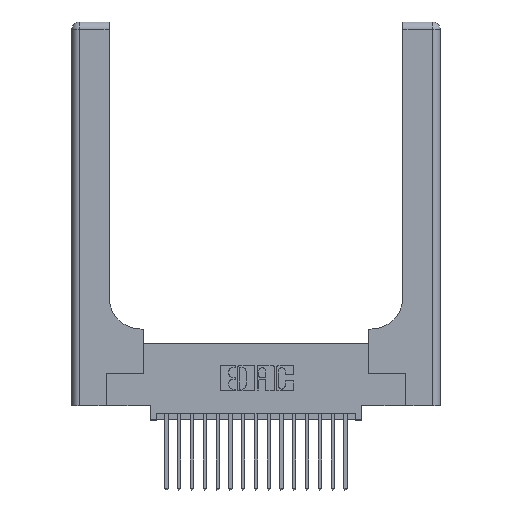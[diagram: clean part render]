
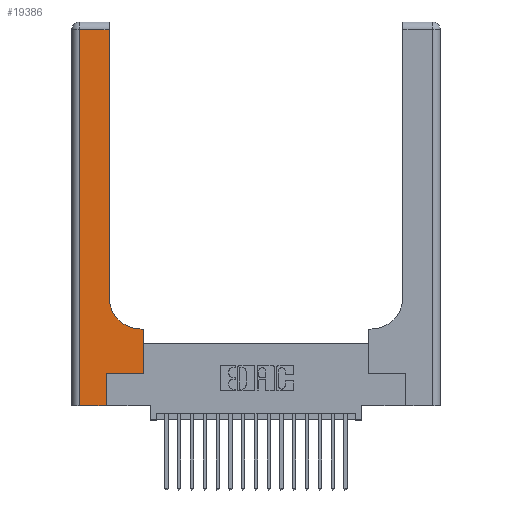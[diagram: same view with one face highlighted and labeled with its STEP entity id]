
A CAD part, top view. The second image highlights one B-rep face of the part: STEP entity #19386.
In plain terms, the highlighted planar face has unit normal (0, 0, 1).
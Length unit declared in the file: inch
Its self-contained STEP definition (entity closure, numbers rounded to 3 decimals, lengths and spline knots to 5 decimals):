
#181 = DIRECTION ( 'NONE',  ( 1., 0., 0. ) ) ;
#705 = LINE ( 'NONE', #16932, #8819 ) ;
#748 = VERTEX_POINT ( 'NONE', #1875 ) ;
#1080 = EDGE_CURVE ( 'NONE', #4931, #9926, #705, .T. ) ;
#1143 = DIRECTION ( 'NONE',  ( 0., 1., 0. ) ) ;
#1218 = ORIENTED_EDGE ( 'NONE', *, *, #17493, .T. ) ;
#1386 = VERTEX_POINT ( 'NONE', #12936 ) ;
#1822 = VECTOR ( 'NONE', #181, 39.37008 ) ;
#1875 = CARTESIAN_POINT ( 'NONE',  ( 0.2915, 2.94, 0.37 ) ) ;
#2050 = LINE ( 'NONE', #8583, #17561 ) ;
#3227 = EDGE_CURVE ( 'NONE', #7083, #1386, #7642, .T. ) ;
#3342 = VECTOR ( 'NONE', #7728, 39.37008 ) ;
#3716 = AXIS2_PLACEMENT_3D ( 'NONE', #9693, #17156, #11349 ) ;
#3732 = LINE ( 'NONE', #12469, #11854 ) ;
#3959 = AXIS2_PLACEMENT_3D ( 'NONE', #14733, #5091, #16300 ) ;
#4046 = CIRCLE ( 'NONE', #3959, 0.25 ) ;
#4320 = CARTESIAN_POINT ( 'NONE',  ( 0.2915, 3., 0.37 ) ) ;
#4522 = VERTEX_POINT ( 'NONE', #17471 ) ;
#4611 = ORIENTED_EDGE ( 'NONE', *, *, #19188, .T. ) ;
#4773 = CARTESIAN_POINT ( 'NONE',  ( 0., 2.94, 0.37 ) ) ;
#4931 = VERTEX_POINT ( 'NONE', #13647 ) ;
#5091 = DIRECTION ( 'NONE',  ( 0., 0., -1. ) ) ;
#5169 = ORIENTED_EDGE ( 'NONE', *, *, #17136, .T. ) ;
#5194 = ORIENTED_EDGE ( 'NONE', *, *, #13864, .T. ) ;
#5975 = LINE ( 'NONE', #16312, #18178 ) ;
#6339 = VERTEX_POINT ( 'NONE', #17138 ) ;
#7083 = VERTEX_POINT ( 'NONE', #10595 ) ;
#7498 = VECTOR ( 'NONE', #17559, 39.37008 ) ;
#7582 = DIRECTION ( 'NONE',  ( 0., 1., 0. ) ) ;
#7642 = LINE ( 'NONE', #8722, #3342 ) ;
#7728 = DIRECTION ( 'NONE',  ( 1., 0., 0. ) ) ;
#8287 = VERTEX_POINT ( 'NONE', #20000 ) ;
#8354 = DIRECTION ( 'NONE',  ( 0., -1., 0. ) ) ;
#8583 = CARTESIAN_POINT ( 'NONE',  ( 0.269, 0., 0.37 ) ) ;
#8722 = CARTESIAN_POINT ( 'NONE',  ( 0., 0., 0.37 ) ) ;
#8819 = VECTOR ( 'NONE', #16775, 39.37008 ) ;
#9693 = CARTESIAN_POINT ( 'NONE',  ( 0., 3., 0.37 ) ) ;
#9926 = VERTEX_POINT ( 'NONE', #19060 ) ;
#10595 = CARTESIAN_POINT ( 'NONE',  ( 0.06, 0., 0.37 ) ) ;
#11143 = EDGE_CURVE ( 'NONE', #748, #8287, #20186, .T. ) ;
#11230 = VECTOR ( 'NONE', #1143, 39.37008 ) ;
#11349 = DIRECTION ( 'NONE',  ( -1., 0., 0. ) ) ;
#11565 = CARTESIAN_POINT ( 'NONE',  ( 0.269, 0.25, 0.37 ) ) ;
#11718 = EDGE_CURVE ( 'NONE', #8287, #7083, #5975, .T. ) ;
#11854 = VECTOR ( 'NONE', #7582, 39.37008 ) ;
#11867 = DIRECTION ( 'NONE',  ( 0., 1., 0. ) ) ;
#11878 = FACE_OUTER_BOUND ( 'NONE', #16719, .T. ) ;
#12469 = CARTESIAN_POINT ( 'NONE',  ( 0.5585, 0.25, 0.37 ) ) ;
#12810 = ORIENTED_EDGE ( 'NONE', *, *, #11143, .T. ) ;
#12936 = CARTESIAN_POINT ( 'NONE',  ( 0.269, 0., 0.37 ) ) ;
#13647 = CARTESIAN_POINT ( 'NONE',  ( 0.5585, 0.6, 0.37 ) ) ;
#13864 = EDGE_CURVE ( 'NONE', #4522, #6339, #14671, .T. ) ;
#13956 = ORIENTED_EDGE ( 'NONE', *, *, #11718, .T. ) ;
#14671 = LINE ( 'NONE', #11565, #1822 ) ;
#14733 = CARTESIAN_POINT ( 'NONE',  ( 0.5415, 0.85, 0.37 ) ) ;
#15617 = EDGE_CURVE ( 'NONE', #19931, #748, #20105, .T. ) ;
#16300 = DIRECTION ( 'NONE',  ( 1., 0., 0. ) ) ;
#16312 = CARTESIAN_POINT ( 'NONE',  ( 0.06, 3., 0.37 ) ) ;
#16395 = ORIENTED_EDGE ( 'NONE', *, *, #15617, .T. ) ;
#16719 = EDGE_LOOP ( 'NONE', ( #16395, #12810, #13956, #17787, #5169, #5194, #4611, #19234, #1218 ) ) ;
#16775 = DIRECTION ( 'NONE',  ( -1., 0., 0. ) ) ;
#16932 = CARTESIAN_POINT ( 'NONE',  ( 0.2915, 0.6, 0.37 ) ) ;
#17136 = EDGE_CURVE ( 'NONE', #1386, #4522, #2050, .T. ) ;
#17138 = CARTESIAN_POINT ( 'NONE',  ( 0.5585, 0.25, 0.37 ) ) ;
#17156 = DIRECTION ( 'NONE',  ( 0., 0., -1. ) ) ;
#17437 = CARTESIAN_POINT ( 'NONE',  ( 0.2915, 0.85, 0.37 ) ) ;
#17471 = CARTESIAN_POINT ( 'NONE',  ( 0.269, 0.25, 0.37 ) ) ;
#17493 = EDGE_CURVE ( 'NONE', #9926, #19931, #4046, .T. ) ;
#17559 = DIRECTION ( 'NONE',  ( -1., 0., 0. ) ) ;
#17561 = VECTOR ( 'NONE', #11867, 39.37008 ) ;
#17590 = PLANE ( 'NONE',  #3716 ) ;
#17787 = ORIENTED_EDGE ( 'NONE', *, *, #3227, .T. ) ;
#18178 = VECTOR ( 'NONE', #8354, 39.37008 ) ;
#19060 = CARTESIAN_POINT ( 'NONE',  ( 0.5415, 0.6, 0.37 ) ) ;
#19188 = EDGE_CURVE ( 'NONE', #6339, #4931, #3732, .T. ) ;
#19234 = ORIENTED_EDGE ( 'NONE', *, *, #1080, .T. ) ;
#19386 = ADVANCED_FACE ( 'NONE', ( #11878 ), #17590, .F. ) ;
#19931 = VERTEX_POINT ( 'NONE', #17437 ) ;
#20000 = CARTESIAN_POINT ( 'NONE',  ( 0.06, 2.94, 0.37 ) ) ;
#20105 = LINE ( 'NONE', #4320, #11230 ) ;
#20186 = LINE ( 'NONE', #4773, #7498 ) ;
